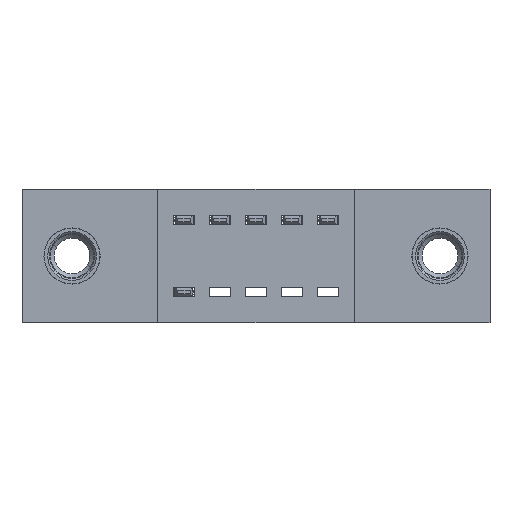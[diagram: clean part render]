
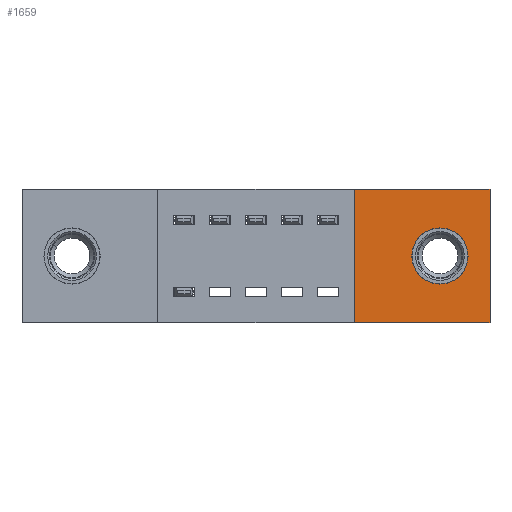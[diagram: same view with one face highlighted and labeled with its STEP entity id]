
A CAD part, front view. The second image highlights one B-rep face of the part: STEP entity #1659.
In plain terms, the highlighted planar face has unit normal (0, -1, 0).
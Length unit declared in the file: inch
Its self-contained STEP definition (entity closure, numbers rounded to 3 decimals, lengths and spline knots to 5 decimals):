
#96 = LINE ( 'NONE', #8505, #7170 ) ;
#131 = EDGE_LOOP ( 'NONE', ( #1125, #887, #3619, #2706 ) ) ;
#188 = VERTEX_POINT ( 'NONE', #4394 ) ;
#321 = EDGE_CURVE ( 'NONE', #3353, #3773, #5301, .T. ) ;
#358 = AXIS2_PLACEMENT_3D ( 'NONE', #6687, #3200, #7684 ) ;
#584 = PLANE ( 'NONE',  #358 ) ;
#768 = FACE_OUTER_BOUND ( 'NONE', #131, .T. ) ;
#887 = ORIENTED_EDGE ( 'NONE', *, *, #321, .F. ) ;
#944 = CIRCLE ( 'NONE', #4317, 0.078 ) ;
#1117 = CARTESIAN_POINT ( 'NONE',  ( 0., 0., -0.37 ) ) ;
#1125 = ORIENTED_EDGE ( 'NONE', *, *, #1734, .F. ) ;
#1352 = VERTEX_POINT ( 'NONE', #4193 ) ;
#1455 = AXIS2_PLACEMENT_3D ( 'NONE', #8000, #4031, #8630 ) ;
#1605 = CARTESIAN_POINT ( 'NONE',  ( 1.3, 0., 0. ) ) ;
#1659 = ADVANCED_FACE ( 'NONE', ( #6018, #768 ), #584, .T. ) ;
#1734 = EDGE_CURVE ( 'NONE', #3773, #2309, #96, .T. ) ;
#1771 = VECTOR ( 'NONE', #2206, 39.37008 ) ;
#1772 = EDGE_LOOP ( 'NONE', ( #3627, #4796 ) ) ;
#2206 = DIRECTION ( 'NONE',  ( 1., 0., 0. ) ) ;
#2267 = LINE ( 'NONE', #1605, #5696 ) ;
#2298 = DIRECTION ( 'NONE',  ( 0., 0., -1. ) ) ;
#2309 = VERTEX_POINT ( 'NONE', #3342 ) ;
#2555 = CARTESIAN_POINT ( 'NONE',  ( 1.3, 0., -0.37 ) ) ;
#2706 = ORIENTED_EDGE ( 'NONE', *, *, #5117, .F. ) ;
#3200 = DIRECTION ( 'NONE',  ( 0., -1., 0. ) ) ;
#3342 = CARTESIAN_POINT ( 'NONE',  ( 0.923, 0., 0. ) ) ;
#3353 = VERTEX_POINT ( 'NONE', #2555 ) ;
#3619 = ORIENTED_EDGE ( 'NONE', *, *, #7125, .F. ) ;
#3627 = ORIENTED_EDGE ( 'NONE', *, *, #8550, .T. ) ;
#3773 = VERTEX_POINT ( 'NONE', #6998 ) ;
#4031 = DIRECTION ( 'NONE',  ( 0., 1., 0. ) ) ;
#4124 = DIRECTION ( 'NONE',  ( 0., 1., 0. ) ) ;
#4193 = CARTESIAN_POINT ( 'NONE',  ( 1.161, 0., -0.107 ) ) ;
#4317 = AXIS2_PLACEMENT_3D ( 'NONE', #8084, #4124, #8716 ) ;
#4394 = CARTESIAN_POINT ( 'NONE',  ( 1.161, 0., -0.263 ) ) ;
#4796 = ORIENTED_EDGE ( 'NONE', *, *, #6770, .T. ) ;
#4902 = VERTEX_POINT ( 'NONE', #7367 ) ;
#5090 = VECTOR ( 'NONE', #5922, 39.37008 ) ;
#5117 = EDGE_CURVE ( 'NONE', #2309, #4902, #5428, .T. ) ;
#5301 = LINE ( 'NONE', #1117, #5090 ) ;
#5428 = LINE ( 'NONE', #7573, #1771 ) ;
#5696 = VECTOR ( 'NONE', #2298, 39.37008 ) ;
#5922 = DIRECTION ( 'NONE',  ( -1., 0., 0. ) ) ;
#6018 = FACE_BOUND ( 'NONE', #1772, .T. ) ;
#6507 = DIRECTION ( 'NONE',  ( 0., 0., 1. ) ) ;
#6687 = CARTESIAN_POINT ( 'NONE',  ( 0., 0., -0.37 ) ) ;
#6770 = EDGE_CURVE ( 'NONE', #188, #1352, #7065, .T. ) ;
#6998 = CARTESIAN_POINT ( 'NONE',  ( 0.923, 0., -0.37 ) ) ;
#7065 = CIRCLE ( 'NONE', #1455, 0.078 ) ;
#7125 = EDGE_CURVE ( 'NONE', #4902, #3353, #2267, .T. ) ;
#7170 = VECTOR ( 'NONE', #6507, 39.37008 ) ;
#7367 = CARTESIAN_POINT ( 'NONE',  ( 1.3, 0., 0. ) ) ;
#7573 = CARTESIAN_POINT ( 'NONE',  ( 0., 0., 0. ) ) ;
#7684 = DIRECTION ( 'NONE',  ( 0., 0., -1. ) ) ;
#8000 = CARTESIAN_POINT ( 'NONE',  ( 1.161, 0., -0.185 ) ) ;
#8084 = CARTESIAN_POINT ( 'NONE',  ( 1.161, 0., -0.185 ) ) ;
#8505 = CARTESIAN_POINT ( 'NONE',  ( 0.923, 0., -0.37 ) ) ;
#8550 = EDGE_CURVE ( 'NONE', #1352, #188, #944, .T. ) ;
#8630 = DIRECTION ( 'NONE',  ( 0., 0., -1. ) ) ;
#8716 = DIRECTION ( 'NONE',  ( 0., 0., -1. ) ) ;
